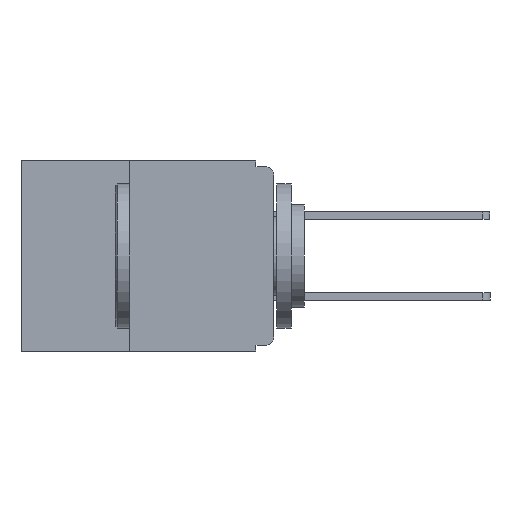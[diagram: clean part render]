
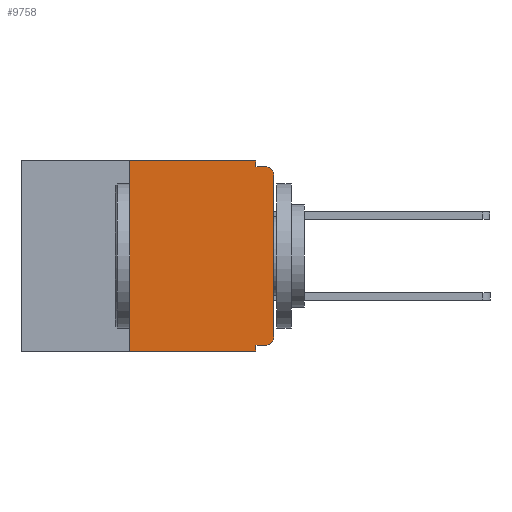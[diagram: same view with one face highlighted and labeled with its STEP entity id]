
A CAD part, left-side view. The second image highlights one B-rep face of the part: STEP entity #9758.
In plain terms, the highlighted planar face has unit normal (-1, 0, 0).
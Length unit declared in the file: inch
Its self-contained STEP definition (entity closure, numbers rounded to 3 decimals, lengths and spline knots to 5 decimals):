
#134 = DIRECTION ( 'NONE',  ( 0., 0., 1. ) ) ;
#144 = VECTOR ( 'NONE', #8062, 39.37008 ) ;
#151 = CARTESIAN_POINT ( 'NONE',  ( 0., 0.25, -0.33 ) ) ;
#206 = LINE ( 'NONE', #16555, #14616 ) ;
#327 = EDGE_CURVE ( 'NONE', #10539, #1458, #206, .T. ) ;
#592 = LINE ( 'NONE', #12316, #144 ) ;
#1015 = CIRCLE ( 'NONE', #7017, 0.015 ) ;
#1458 = VERTEX_POINT ( 'NONE', #4912 ) ;
#1497 = CARTESIAN_POINT ( 'NONE',  ( 0., 0.015, -0.32 ) ) ;
#1614 = FACE_OUTER_BOUND ( 'NONE', #5272, .T. ) ;
#2012 = EDGE_CURVE ( 'NONE', #5561, #7074, #16300, .T. ) ;
#2014 = DIRECTION ( 'NONE',  ( 0., -1., 0. ) ) ;
#2174 = VECTOR ( 'NONE', #16281, 39.37008 ) ;
#2218 = DIRECTION ( 'NONE',  ( -1., 0., 0. ) ) ;
#2232 = ORIENTED_EDGE ( 'NONE', *, *, #4471, .F. ) ;
#2393 = ORIENTED_EDGE ( 'NONE', *, *, #6592, .F. ) ;
#2730 = EDGE_CURVE ( 'NONE', #9771, #7074, #10382, .T. ) ;
#2858 = LINE ( 'NONE', #4272, #6787 ) ;
#3275 = CARTESIAN_POINT ( 'NONE',  ( 0., 0.031, 0. ) ) ;
#3603 = CARTESIAN_POINT ( 'NONE',  ( 0., 0.25, 0. ) ) ;
#3612 = ORIENTED_EDGE ( 'NONE', *, *, #2012, .T. ) ;
#3614 = ORIENTED_EDGE ( 'NONE', *, *, #2730, .F. ) ;
#4096 = VECTOR ( 'NONE', #134, 39.37008 ) ;
#4160 = CARTESIAN_POINT ( 'NONE',  ( 0., 0.437, 0. ) ) ;
#4272 = CARTESIAN_POINT ( 'NONE',  ( 0., 0., 0. ) ) ;
#4471 = EDGE_CURVE ( 'NONE', #17688, #10539, #14927, .T. ) ;
#4529 = VERTEX_POINT ( 'NONE', #8284 ) ;
#4864 = DIRECTION ( 'NONE',  ( -1., 0., 0. ) ) ;
#4912 = CARTESIAN_POINT ( 'NONE',  ( 0., 0.031, -0.01 ) ) ;
#5272 = EDGE_LOOP ( 'NONE', ( #12897, #12934, #14946, #15354, #2232, #2393, #3612, #3614, #6583, #8231 ) ) ;
#5561 = VERTEX_POINT ( 'NONE', #10895 ) ;
#5651 = DIRECTION ( 'NONE',  ( 0., 0., -1. ) ) ;
#5844 = CARTESIAN_POINT ( 'NONE',  ( 0., 0.015, -0.01 ) ) ;
#5897 = VERTEX_POINT ( 'NONE', #7413 ) ;
#6035 = CARTESIAN_POINT ( 'NONE',  ( 0., 0.031, -0.33 ) ) ;
#6519 = LINE ( 'NONE', #9031, #17335 ) ;
#6583 = ORIENTED_EDGE ( 'NONE', *, *, #17691, .F. ) ;
#6592 = EDGE_CURVE ( 'NONE', #5561, #17688, #15076, .T. ) ;
#6787 = VECTOR ( 'NONE', #14292, 39.37008 ) ;
#6997 = VERTEX_POINT ( 'NONE', #5844 ) ;
#7017 = AXIS2_PLACEMENT_3D ( 'NONE', #13437, #4864, #14836 ) ;
#7074 = VERTEX_POINT ( 'NONE', #6035 ) ;
#7413 = CARTESIAN_POINT ( 'NONE',  ( 0., 0., -0.305 ) ) ;
#7900 = DIRECTION ( 'NONE',  ( 0., 0., -1. ) ) ;
#8062 = DIRECTION ( 'NONE',  ( 0., 1., 0. ) ) ;
#8231 = ORIENTED_EDGE ( 'NONE', *, *, #9545, .T. ) ;
#8284 = CARTESIAN_POINT ( 'NONE',  ( 0., 0., -0.025 ) ) ;
#8373 = VERTEX_POINT ( 'NONE', #1497 ) ;
#8584 = CARTESIAN_POINT ( 'NONE',  ( 0., 0.031, -0.32 ) ) ;
#9031 = CARTESIAN_POINT ( 'NONE',  ( 0., 0., -0.01 ) ) ;
#9545 = EDGE_CURVE ( 'NONE', #8373, #5897, #16593, .T. ) ;
#9640 = DIRECTION ( 'NONE',  ( 0., -1., 0. ) ) ;
#9758 = ADVANCED_FACE ( 'NONE', ( #1614 ), #9929, .F. ) ;
#9771 = VERTEX_POINT ( 'NONE', #8584 ) ;
#9929 = PLANE ( 'NONE',  #15045 ) ;
#10095 = CARTESIAN_POINT ( 'NONE',  ( 0., 0.437, 0. ) ) ;
#10363 = CARTESIAN_POINT ( 'NONE',  ( 0., 0.031, -0.33 ) ) ;
#10382 = LINE ( 'NONE', #10363, #2174 ) ;
#10458 = DIRECTION ( 'NONE',  ( 0., -1., 0. ) ) ;
#10539 = VERTEX_POINT ( 'NONE', #3275 ) ;
#10895 = CARTESIAN_POINT ( 'NONE',  ( 0., 0.25, -0.33 ) ) ;
#10936 = CARTESIAN_POINT ( 'NONE',  ( 0., 0.015, -0.305 ) ) ;
#12316 = CARTESIAN_POINT ( 'NONE',  ( 0., 0., -0.32 ) ) ;
#12389 = DIRECTION ( 'NONE',  ( 0., 0., -1. ) ) ;
#12608 = VECTOR ( 'NONE', #2014, 39.37008 ) ;
#12897 = ORIENTED_EDGE ( 'NONE', *, *, #17973, .T. ) ;
#12934 = ORIENTED_EDGE ( 'NONE', *, *, #13406, .T. ) ;
#13304 = CARTESIAN_POINT ( 'NONE',  ( 0., 0.437, -0.33 ) ) ;
#13406 = EDGE_CURVE ( 'NONE', #4529, #6997, #1015, .T. ) ;
#13437 = CARTESIAN_POINT ( 'NONE',  ( 0., 0.015, -0.025 ) ) ;
#13969 = EDGE_CURVE ( 'NONE', #1458, #6997, #6519, .T. ) ;
#14185 = DIRECTION ( 'NONE',  ( 1., 0., 0. ) ) ;
#14292 = DIRECTION ( 'NONE',  ( 0., 0., 1. ) ) ;
#14478 = VECTOR ( 'NONE', #9640, 39.37008 ) ;
#14616 = VECTOR ( 'NONE', #7900, 39.37008 ) ;
#14836 = DIRECTION ( 'NONE',  ( 0., 0., -1. ) ) ;
#14927 = LINE ( 'NONE', #10095, #14478 ) ;
#14946 = ORIENTED_EDGE ( 'NONE', *, *, #13969, .F. ) ;
#15045 = AXIS2_PLACEMENT_3D ( 'NONE', #4160, #14185, #5651 ) ;
#15076 = LINE ( 'NONE', #151, #4096 ) ;
#15354 = ORIENTED_EDGE ( 'NONE', *, *, #327, .F. ) ;
#16281 = DIRECTION ( 'NONE',  ( 0., 0., -1. ) ) ;
#16300 = LINE ( 'NONE', #13304, #12608 ) ;
#16318 = AXIS2_PLACEMENT_3D ( 'NONE', #10936, #2218, #12389 ) ;
#16555 = CARTESIAN_POINT ( 'NONE',  ( 0., 0.031, 0. ) ) ;
#16593 = CIRCLE ( 'NONE', #16318, 0.015 ) ;
#17335 = VECTOR ( 'NONE', #10458, 39.37008 ) ;
#17688 = VERTEX_POINT ( 'NONE', #3603 ) ;
#17691 = EDGE_CURVE ( 'NONE', #8373, #9771, #592, .T. ) ;
#17973 = EDGE_CURVE ( 'NONE', #5897, #4529, #2858, .T. ) ;
